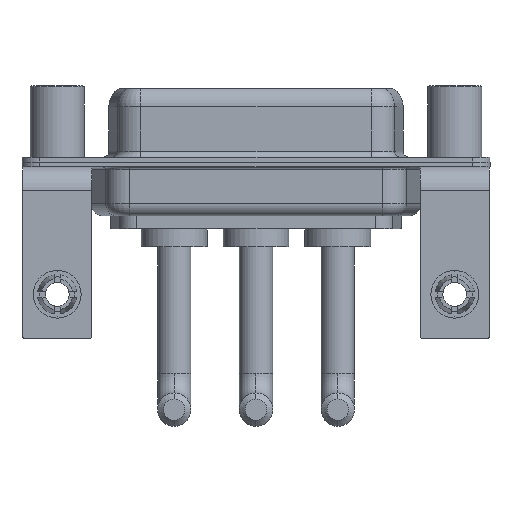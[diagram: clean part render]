
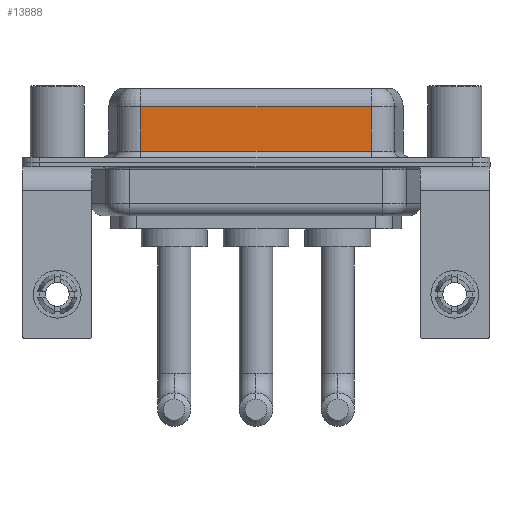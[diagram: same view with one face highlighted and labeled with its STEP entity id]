
A CAD part, front view. The second image highlights one B-rep face of the part: STEP entity #13888.
In plain terms, the highlighted planar face has unit normal (0, -1, 0).
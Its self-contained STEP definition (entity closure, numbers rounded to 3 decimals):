
#42 = DIRECTION ( 'NONE',  ( -1., 0., 0. ) ) ;
#109 = LINE ( 'NONE', #7454, #2733 ) ;
#720 = AXIS2_PLACEMENT_3D ( 'NONE', #12967, #13043, #11696 ) ;
#1625 = EDGE_CURVE ( 'NONE', #6659, #6410, #6238, .T. ) ;
#1906 = LINE ( 'NONE', #7003, #10525 ) ;
#2282 = VECTOR ( 'NONE', #42, 1000. ) ;
#2364 = VERTEX_POINT ( 'NONE', #7419 ) ;
#2733 = VECTOR ( 'NONE', #11513, 1000. ) ;
#3462 = CARTESIAN_POINT ( 'NONE',  ( 26.287, -3.95, 4.65 ) ) ;
#4069 = PLANE ( 'NONE',  #720 ) ;
#4520 = ORIENTED_EDGE ( 'NONE', *, *, #16272, .F. ) ;
#6009 = VERTEX_POINT ( 'NONE', #6987 ) ;
#6238 = LINE ( 'NONE', #11277, #2282 ) ;
#6410 = VERTEX_POINT ( 'NONE', #6482 ) ;
#6482 = CARTESIAN_POINT ( 'NONE',  ( 7.013, -3.95, 4.65 ) ) ;
#6566 = DIRECTION ( 'NONE',  ( 0., 0., -1. ) ) ;
#6659 = VERTEX_POINT ( 'NONE', #3462 ) ;
#6758 = EDGE_CURVE ( 'NONE', #6009, #2364, #109, .T. ) ;
#6987 = CARTESIAN_POINT ( 'NONE',  ( 7.013, -3.95, 0.9 ) ) ;
#7003 = CARTESIAN_POINT ( 'NONE',  ( 7.013, -3.95, 6.4 ) ) ;
#7419 = CARTESIAN_POINT ( 'NONE',  ( 26.287, -3.95, 0.9 ) ) ;
#7454 = CARTESIAN_POINT ( 'NONE',  ( 26.287, -3.95, 0.9 ) ) ;
#8801 = CARTESIAN_POINT ( 'NONE',  ( 26.287, -3.95, 6.4 ) ) ;
#9243 = VECTOR ( 'NONE', #6566, 1000. ) ;
#9706 = EDGE_LOOP ( 'NONE', ( #4520, #14377, #14108, #10621 ) ) ;
#10525 = VECTOR ( 'NONE', #12067, 1000. ) ;
#10621 = ORIENTED_EDGE ( 'NONE', *, *, #6758, .T. ) ;
#11277 = CARTESIAN_POINT ( 'NONE',  ( 26.287, -3.95, 4.65 ) ) ;
#11513 = DIRECTION ( 'NONE',  ( 1., 0., 0. ) ) ;
#11532 = FACE_OUTER_BOUND ( 'NONE', #9706, .T. ) ;
#11696 = DIRECTION ( 'NONE',  ( 0., 0., 1. ) ) ;
#12067 = DIRECTION ( 'NONE',  ( 0., 0., -1. ) ) ;
#12967 = CARTESIAN_POINT ( 'NONE',  ( 26.287, -3.95, 6.4 ) ) ;
#13043 = DIRECTION ( 'NONE',  ( 0., 1., 0. ) ) ;
#13145 = EDGE_CURVE ( 'NONE', #6410, #6009, #1906, .T. ) ;
#13888 = ADVANCED_FACE ( 'NONE', ( #11532 ), #4069, .F. ) ;
#14108 = ORIENTED_EDGE ( 'NONE', *, *, #13145, .T. ) ;
#14377 = ORIENTED_EDGE ( 'NONE', *, *, #1625, .T. ) ;
#15222 = LINE ( 'NONE', #8801, #9243 ) ;
#16272 = EDGE_CURVE ( 'NONE', #6659, #2364, #15222, .T. ) ;
